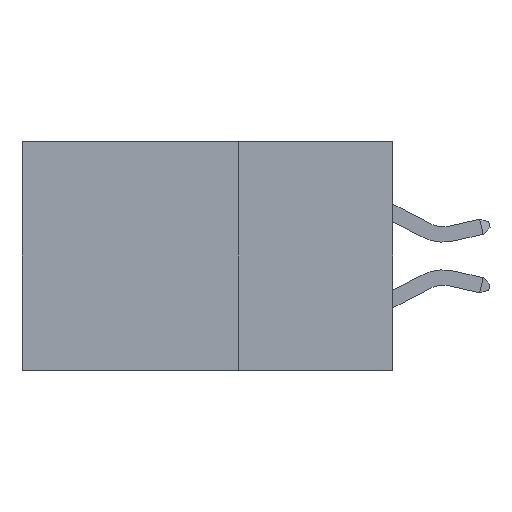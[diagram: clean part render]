
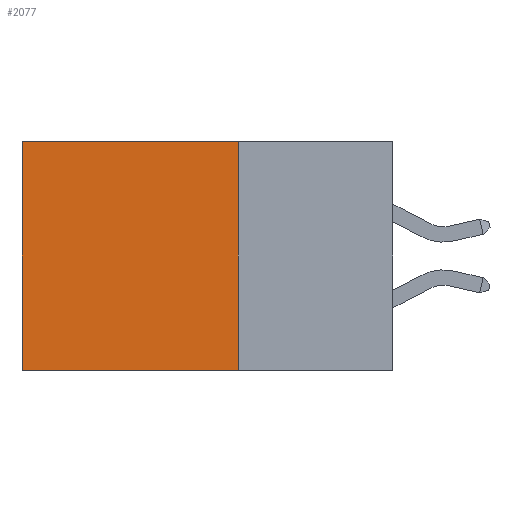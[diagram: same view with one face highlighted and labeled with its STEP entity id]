
A CAD part, left-side view. The second image highlights one B-rep face of the part: STEP entity #2077.
In plain terms, the highlighted planar face has unit normal (-1, 0, 0).
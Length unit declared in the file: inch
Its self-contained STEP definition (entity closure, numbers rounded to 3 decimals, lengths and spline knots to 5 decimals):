
#86 = EDGE_LOOP ( 'NONE', ( #9169, #1042, #6587, #3710 ) ) ;
#339 = VERTEX_POINT ( 'NONE', #733 ) ;
#472 = LINE ( 'NONE', #7108, #4017 ) ;
#581 = LINE ( 'NONE', #6581, #3892 ) ;
#733 = CARTESIAN_POINT ( 'NONE',  ( 0.2875, 0.6, 0. ) ) ;
#778 = CARTESIAN_POINT ( 'NONE',  ( 0.2875, 0.25, 0. ) ) ;
#1042 = ORIENTED_EDGE ( 'NONE', *, *, #4025, .F. ) ;
#1272 = CARTESIAN_POINT ( 'NONE',  ( 0.2875, 0.25, 0. ) ) ;
#1711 = CARTESIAN_POINT ( 'NONE',  ( 0.2875, 0.25, 0. ) ) ;
#1944 = AXIS2_PLACEMENT_3D ( 'NONE', #778, #2244, #4458 ) ;
#1963 = DIRECTION ( 'NONE',  ( 0., 1., 0. ) ) ;
#2077 = ADVANCED_FACE ( 'NONE', ( #2537 ), #7479, .F. ) ;
#2244 = DIRECTION ( 'NONE',  ( 1., 0., 0. ) ) ;
#2528 = DIRECTION ( 'NONE',  ( 0., 0., -1. ) ) ;
#2537 = FACE_OUTER_BOUND ( 'NONE', #86, .T. ) ;
#3603 = VERTEX_POINT ( 'NONE', #1711 ) ;
#3710 = ORIENTED_EDGE ( 'NONE', *, *, #7934, .T. ) ;
#3892 = VECTOR ( 'NONE', #7333, 39.37008 ) ;
#4017 = VECTOR ( 'NONE', #2528, 39.37008 ) ;
#4025 = EDGE_CURVE ( 'NONE', #4051, #5443, #4177, .T. ) ;
#4051 = VERTEX_POINT ( 'NONE', #6175 ) ;
#4177 = LINE ( 'NONE', #7013, #9145 ) ;
#4404 = CARTESIAN_POINT ( 'NONE',  ( 0.2875, 0.6, -0.37 ) ) ;
#4458 = DIRECTION ( 'NONE',  ( 0., 0., -1. ) ) ;
#5442 = DIRECTION ( 'NONE',  ( 0., 1., 0. ) ) ;
#5443 = VERTEX_POINT ( 'NONE', #4404 ) ;
#6175 = CARTESIAN_POINT ( 'NONE',  ( 0.2875, 0.25, -0.37 ) ) ;
#6581 = CARTESIAN_POINT ( 'NONE',  ( 0.2875, 0.25, 0. ) ) ;
#6587 = ORIENTED_EDGE ( 'NONE', *, *, #7583, .F. ) ;
#7013 = CARTESIAN_POINT ( 'NONE',  ( 0.2875, 0.25, -0.37 ) ) ;
#7108 = CARTESIAN_POINT ( 'NONE',  ( 0.2875, 0.6, 0. ) ) ;
#7333 = DIRECTION ( 'NONE',  ( 0., 0., -1. ) ) ;
#7459 = LINE ( 'NONE', #1272, #9712 ) ;
#7479 = PLANE ( 'NONE',  #1944 ) ;
#7583 = EDGE_CURVE ( 'NONE', #3603, #4051, #581, .T. ) ;
#7822 = EDGE_CURVE ( 'NONE', #339, #5443, #472, .T. ) ;
#7934 = EDGE_CURVE ( 'NONE', #3603, #339, #7459, .T. ) ;
#9145 = VECTOR ( 'NONE', #5442, 39.37008 ) ;
#9169 = ORIENTED_EDGE ( 'NONE', *, *, #7822, .T. ) ;
#9712 = VECTOR ( 'NONE', #1963, 39.37008 ) ;
